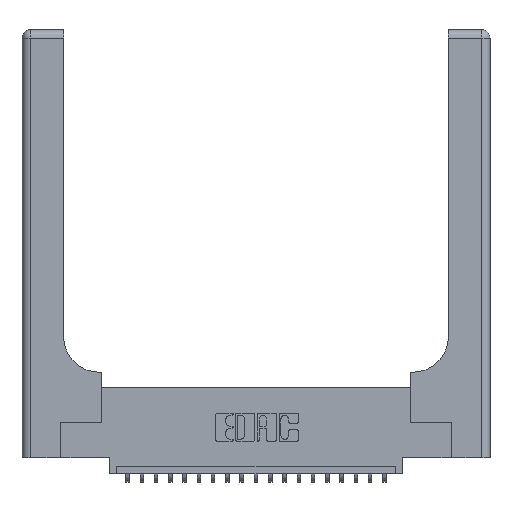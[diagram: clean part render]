
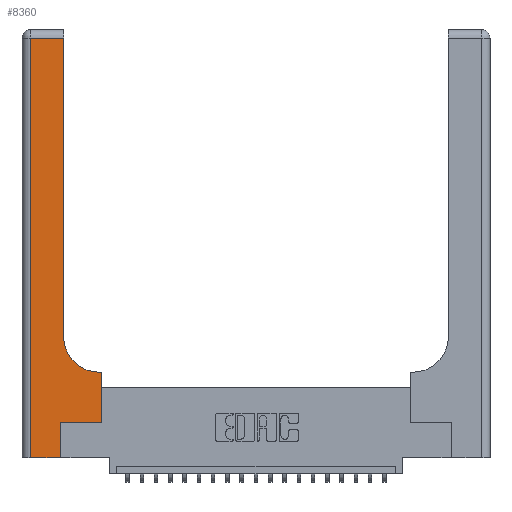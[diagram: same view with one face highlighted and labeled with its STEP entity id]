
A CAD part, top view. The second image highlights one B-rep face of the part: STEP entity #8360.
In plain terms, the highlighted planar face has unit normal (0, 0, 1).
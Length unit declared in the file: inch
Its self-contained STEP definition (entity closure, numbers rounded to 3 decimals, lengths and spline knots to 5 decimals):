
#164 = CARTESIAN_POINT ( 'NONE',  ( 0.2915, 2.94, 0.37 ) ) ;
#714 = VERTEX_POINT ( 'NONE', #9217 ) ;
#882 = EDGE_CURVE ( 'NONE', #15116, #7672, #4965, .T. ) ;
#1495 = ORIENTED_EDGE ( 'NONE', *, *, #18880, .T. ) ;
#1871 = CARTESIAN_POINT ( 'NONE',  ( 0.5585, 0.25, 0.37 ) ) ;
#2289 = CARTESIAN_POINT ( 'NONE',  ( 0.2915, 3., 0.37 ) ) ;
#2403 = VECTOR ( 'NONE', #16057, 39.37008 ) ;
#2950 = VERTEX_POINT ( 'NONE', #16868 ) ;
#3079 = CARTESIAN_POINT ( 'NONE',  ( 0.269, 0.25, 0.37 ) ) ;
#3269 = VERTEX_POINT ( 'NONE', #3079 ) ;
#3576 = CARTESIAN_POINT ( 'NONE',  ( 0.2915, 0.6, 0.37 ) ) ;
#4577 = ORIENTED_EDGE ( 'NONE', *, *, #9266, .T. ) ;
#4601 = LINE ( 'NONE', #7124, #2403 ) ;
#4965 = LINE ( 'NONE', #1871, #12481 ) ;
#5027 = FACE_OUTER_BOUND ( 'NONE', #20078, .T. ) ;
#5380 = ORIENTED_EDGE ( 'NONE', *, *, #6101, .T. ) ;
#5922 = CARTESIAN_POINT ( 'NONE',  ( 0.5415, 0.6, 0.37 ) ) ;
#6016 = AXIS2_PLACEMENT_3D ( 'NONE', #16408, #16485, #14569 ) ;
#6101 = EDGE_CURVE ( 'NONE', #2950, #714, #14765, .T. ) ;
#6886 = CARTESIAN_POINT ( 'NONE',  ( 0.269, 0., 0.37 ) ) ;
#6930 = VECTOR ( 'NONE', #21588, 39.37008 ) ;
#7124 = CARTESIAN_POINT ( 'NONE',  ( 0.269, 0.25, 0.37 ) ) ;
#7406 = LINE ( 'NONE', #2289, #12662 ) ;
#7672 = VERTEX_POINT ( 'NONE', #12539 ) ;
#8360 = ADVANCED_FACE ( 'NONE', ( #5027 ), #12736, .F. ) ;
#8432 = DIRECTION ( 'NONE',  ( 0., 0., -1. ) ) ;
#8590 = DIRECTION ( 'NONE',  ( 0., 1., 0. ) ) ;
#9217 = CARTESIAN_POINT ( 'NONE',  ( 0.269, 0., 0.37 ) ) ;
#9266 = EDGE_CURVE ( 'NONE', #13643, #2950, #11675, .T. ) ;
#10151 = CARTESIAN_POINT ( 'NONE',  ( 0.06, 2.94, 0.37 ) ) ;
#10183 = EDGE_CURVE ( 'NONE', #11962, #21904, #12696, .T. ) ;
#10463 = EDGE_CURVE ( 'NONE', #22219, #13643, #11800, .T. ) ;
#11553 = EDGE_CURVE ( 'NONE', #7672, #11962, #15689, .T. ) ;
#11675 = LINE ( 'NONE', #18100, #6930 ) ;
#11800 = LINE ( 'NONE', #13087, #15328 ) ;
#11962 = VERTEX_POINT ( 'NONE', #5922 ) ;
#12481 = VECTOR ( 'NONE', #8590, 39.37008 ) ;
#12539 = CARTESIAN_POINT ( 'NONE',  ( 0.5585, 0.6, 0.37 ) ) ;
#12662 = VECTOR ( 'NONE', #19856, 39.37008 ) ;
#12696 = CIRCLE ( 'NONE', #19302, 0.25 ) ;
#12736 = PLANE ( 'NONE',  #6016 ) ;
#13087 = CARTESIAN_POINT ( 'NONE',  ( 0., 2.94, 0.37 ) ) ;
#13222 = CARTESIAN_POINT ( 'NONE',  ( 0.5585, 0.25, 0.37 ) ) ;
#13643 = VERTEX_POINT ( 'NONE', #10151 ) ;
#14188 = DIRECTION ( 'NONE',  ( -1., 0., 0. ) ) ;
#14448 = ORIENTED_EDGE ( 'NONE', *, *, #18248, .T. ) ;
#14569 = DIRECTION ( 'NONE',  ( -1., 0., 0. ) ) ;
#14765 = LINE ( 'NONE', #20607, #15310 ) ;
#14783 = EDGE_CURVE ( 'NONE', #714, #3269, #17514, .T. ) ;
#15116 = VERTEX_POINT ( 'NONE', #13222 ) ;
#15159 = CARTESIAN_POINT ( 'NONE',  ( 0.2915, 0.85, 0.37 ) ) ;
#15271 = ORIENTED_EDGE ( 'NONE', *, *, #11553, .T. ) ;
#15310 = VECTOR ( 'NONE', #22358, 39.37008 ) ;
#15328 = VECTOR ( 'NONE', #16605, 39.37008 ) ;
#15689 = LINE ( 'NONE', #3576, #16814 ) ;
#15704 = ORIENTED_EDGE ( 'NONE', *, *, #10463, .T. ) ;
#16057 = DIRECTION ( 'NONE',  ( 1., 0., 0. ) ) ;
#16355 = ORIENTED_EDGE ( 'NONE', *, *, #882, .T. ) ;
#16408 = CARTESIAN_POINT ( 'NONE',  ( 0., 3., 0.37 ) ) ;
#16485 = DIRECTION ( 'NONE',  ( 0., 0., -1. ) ) ;
#16605 = DIRECTION ( 'NONE',  ( -1., 0., 0. ) ) ;
#16814 = VECTOR ( 'NONE', #14188, 39.37008 ) ;
#16868 = CARTESIAN_POINT ( 'NONE',  ( 0.06, 0., 0.37 ) ) ;
#17514 = LINE ( 'NONE', #6886, #18065 ) ;
#18065 = VECTOR ( 'NONE', #19209, 39.37008 ) ;
#18100 = CARTESIAN_POINT ( 'NONE',  ( 0.06, 3., 0.37 ) ) ;
#18248 = EDGE_CURVE ( 'NONE', #21904, #22219, #7406, .T. ) ;
#18880 = EDGE_CURVE ( 'NONE', #3269, #15116, #4601, .T. ) ;
#19044 = ORIENTED_EDGE ( 'NONE', *, *, #10183, .T. ) ;
#19209 = DIRECTION ( 'NONE',  ( 0., 1., 0. ) ) ;
#19302 = AXIS2_PLACEMENT_3D ( 'NONE', #22407, #8432, #22328 ) ;
#19856 = DIRECTION ( 'NONE',  ( 0., 1., 0. ) ) ;
#20078 = EDGE_LOOP ( 'NONE', ( #14448, #15704, #4577, #5380, #21435, #1495, #16355, #15271, #19044 ) ) ;
#20607 = CARTESIAN_POINT ( 'NONE',  ( 0., 0., 0.37 ) ) ;
#21435 = ORIENTED_EDGE ( 'NONE', *, *, #14783, .T. ) ;
#21588 = DIRECTION ( 'NONE',  ( 0., -1., 0. ) ) ;
#21904 = VERTEX_POINT ( 'NONE', #15159 ) ;
#22219 = VERTEX_POINT ( 'NONE', #164 ) ;
#22328 = DIRECTION ( 'NONE',  ( 1., 0., 0. ) ) ;
#22358 = DIRECTION ( 'NONE',  ( 1., 0., 0. ) ) ;
#22407 = CARTESIAN_POINT ( 'NONE',  ( 0.5415, 0.85, 0.37 ) ) ;
